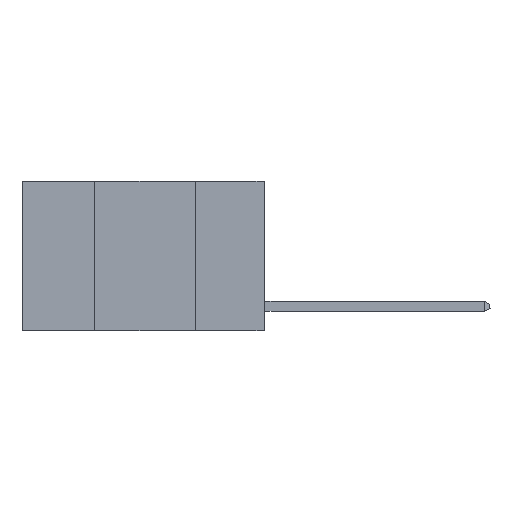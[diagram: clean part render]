
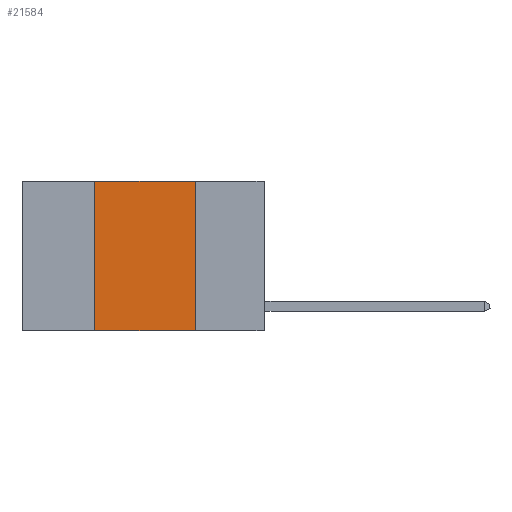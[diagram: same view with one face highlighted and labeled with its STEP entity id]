
A CAD part, left-side view. The second image highlights one B-rep face of the part: STEP entity #21584.
In plain terms, the highlighted planar face has unit normal (-1, 0, 0).
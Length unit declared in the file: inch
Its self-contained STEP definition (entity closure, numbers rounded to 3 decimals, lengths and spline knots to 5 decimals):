
#597 = DIRECTION ( 'NONE',  ( 0., 0., 1. ) ) ;
#871 = PLANE ( 'NONE',  #21761 ) ;
#1930 = CARTESIAN_POINT ( 'NONE',  ( 0., 0.17, 0. ) ) ;
#1989 = DIRECTION ( 'NONE',  ( 0., -1., 0. ) ) ;
#2111 = VECTOR ( 'NONE', #1989, 39.37008 ) ;
#4246 = ORIENTED_EDGE ( 'NONE', *, *, #4254, .T. ) ;
#4254 = EDGE_CURVE ( 'NONE', #15522, #8370, #20733, .T. ) ;
#4369 = CARTESIAN_POINT ( 'NONE',  ( 0., 0.6, 0. ) ) ;
#4862 = VERTEX_POINT ( 'NONE', #1930 ) ;
#5565 = LINE ( 'NONE', #20904, #7129 ) ;
#5847 = DIRECTION ( 'NONE',  ( 1., 0., 0. ) ) ;
#5953 = DIRECTION ( 'NONE',  ( 0., 0., -1. ) ) ;
#6798 = ORIENTED_EDGE ( 'NONE', *, *, #7662, .F. ) ;
#7129 = VECTOR ( 'NONE', #597, 39.37008 ) ;
#7662 = EDGE_CURVE ( 'NONE', #15522, #11056, #5565, .T. ) ;
#8359 = CARTESIAN_POINT ( 'NONE',  ( 0., 0.42, 0. ) ) ;
#8370 = VERTEX_POINT ( 'NONE', #10813 ) ;
#9796 = LINE ( 'NONE', #14827, #10989 ) ;
#10813 = CARTESIAN_POINT ( 'NONE',  ( 0., 0.17, -0.37 ) ) ;
#10989 = VECTOR ( 'NONE', #16367, 39.37008 ) ;
#11056 = VERTEX_POINT ( 'NONE', #8359 ) ;
#11132 = DIRECTION ( 'NONE',  ( 0., -1., 0. ) ) ;
#11185 = EDGE_CURVE ( 'NONE', #4862, #8370, #9796, .T. ) ;
#12479 = CARTESIAN_POINT ( 'NONE',  ( 0., 0.6, 0. ) ) ;
#12864 = EDGE_LOOP ( 'NONE', ( #16220, #16451, #6798, #4246 ) ) ;
#14827 = CARTESIAN_POINT ( 'NONE',  ( 0., 0.17, 0. ) ) ;
#15522 = VERTEX_POINT ( 'NONE', #16275 ) ;
#15987 = EDGE_CURVE ( 'NONE', #11056, #4862, #19599, .T. ) ;
#16220 = ORIENTED_EDGE ( 'NONE', *, *, #11185, .F. ) ;
#16275 = CARTESIAN_POINT ( 'NONE',  ( 0., 0.42, -0.37 ) ) ;
#16367 = DIRECTION ( 'NONE',  ( 0., 0., -1. ) ) ;
#16451 = ORIENTED_EDGE ( 'NONE', *, *, #15987, .F. ) ;
#17607 = FACE_OUTER_BOUND ( 'NONE', #12864, .T. ) ;
#18503 = VECTOR ( 'NONE', #11132, 39.37008 ) ;
#19046 = CARTESIAN_POINT ( 'NONE',  ( 0., 0.6, -0.37 ) ) ;
#19599 = LINE ( 'NONE', #4369, #18503 ) ;
#20733 = LINE ( 'NONE', #19046, #2111 ) ;
#20904 = CARTESIAN_POINT ( 'NONE',  ( 0., 0.42, 0. ) ) ;
#21584 = ADVANCED_FACE ( 'NONE', ( #17607 ), #871, .F. ) ;
#21761 = AXIS2_PLACEMENT_3D ( 'NONE', #12479, #5847, #5953 ) ;
